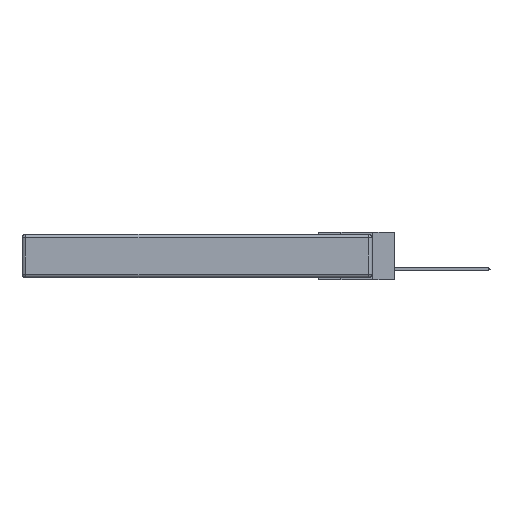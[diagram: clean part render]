
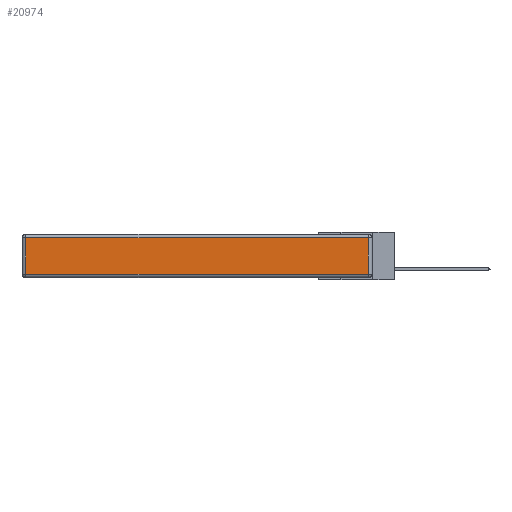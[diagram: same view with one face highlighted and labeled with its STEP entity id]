
A CAD part, left-side view. The second image highlights one B-rep face of the part: STEP entity #20974.
In plain terms, the highlighted planar face has unit normal (-1, 0, 0).
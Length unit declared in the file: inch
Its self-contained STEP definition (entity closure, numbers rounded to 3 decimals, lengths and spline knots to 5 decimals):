
#878 = DIRECTION ( 'NONE',  ( -1., 0., 0. ) ) ;
#2232 = VECTOR ( 'NONE', #6645, 39.37008 ) ;
#3220 = ORIENTED_EDGE ( 'NONE', *, *, #4302, .T. ) ;
#3961 = ORIENTED_EDGE ( 'NONE', *, *, #21326, .T. ) ;
#4302 = EDGE_CURVE ( 'NONE', #27208, #9451, #5658, .T. ) ;
#4752 = DIRECTION ( 'NONE',  ( 0., 0., 1. ) ) ;
#4952 = VECTOR ( 'NONE', #26413, 39.37008 ) ;
#5610 = CARTESIAN_POINT ( 'NONE',  ( 0., 2.72, -0.03 ) ) ;
#5658 = LINE ( 'NONE', #19470, #4952 ) ;
#6645 = DIRECTION ( 'NONE',  ( 0., -1., 0. ) ) ;
#7445 = CARTESIAN_POINT ( 'NONE',  ( 0., 0.03, -0.313 ) ) ;
#7693 = FACE_OUTER_BOUND ( 'NONE', #10273, .T. ) ;
#8343 = VERTEX_POINT ( 'NONE', #7445 ) ;
#9442 = PLANE ( 'NONE',  #22242 ) ;
#9451 = VERTEX_POINT ( 'NONE', #19279 ) ;
#10273 = EDGE_LOOP ( 'NONE', ( #23412, #15494, #3961, #3220 ) ) ;
#10484 = VERTEX_POINT ( 'NONE', #26927 ) ;
#11605 = CARTESIAN_POINT ( 'NONE',  ( 0., 0., -0.343 ) ) ;
#13665 = LINE ( 'NONE', #27721, #2232 ) ;
#14386 = LINE ( 'NONE', #23776, #25421 ) ;
#15455 = DIRECTION ( 'NONE',  ( 0., 1., 0. ) ) ;
#15494 = ORIENTED_EDGE ( 'NONE', *, *, #25500, .T. ) ;
#15729 = CARTESIAN_POINT ( 'NONE',  ( 0., 2.75, -0.03 ) ) ;
#19279 = CARTESIAN_POINT ( 'NONE',  ( 0., 2.72, -0.313 ) ) ;
#19470 = CARTESIAN_POINT ( 'NONE',  ( 0., 2.72, -0.343 ) ) ;
#20974 = ADVANCED_FACE ( 'NONE', ( #7693 ), #9442, .T. ) ;
#21326 = EDGE_CURVE ( 'NONE', #10484, #27208, #22349, .T. ) ;
#21548 = EDGE_CURVE ( 'NONE', #9451, #8343, #13665, .T. ) ;
#22242 = AXIS2_PLACEMENT_3D ( 'NONE', #11605, #878, #26840 ) ;
#22349 = LINE ( 'NONE', #15729, #25372 ) ;
#23412 = ORIENTED_EDGE ( 'NONE', *, *, #21548, .T. ) ;
#23776 = CARTESIAN_POINT ( 'NONE',  ( 0., 0.03, -0.343 ) ) ;
#25372 = VECTOR ( 'NONE', #15455, 39.37008 ) ;
#25421 = VECTOR ( 'NONE', #4752, 39.37008 ) ;
#25500 = EDGE_CURVE ( 'NONE', #8343, #10484, #14386, .T. ) ;
#26413 = DIRECTION ( 'NONE',  ( 0., 0., -1. ) ) ;
#26840 = DIRECTION ( 'NONE',  ( 0., 0., 1. ) ) ;
#26927 = CARTESIAN_POINT ( 'NONE',  ( 0., 0.03, -0.03 ) ) ;
#27208 = VERTEX_POINT ( 'NONE', #5610 ) ;
#27721 = CARTESIAN_POINT ( 'NONE',  ( 0., 0., -0.313 ) ) ;
